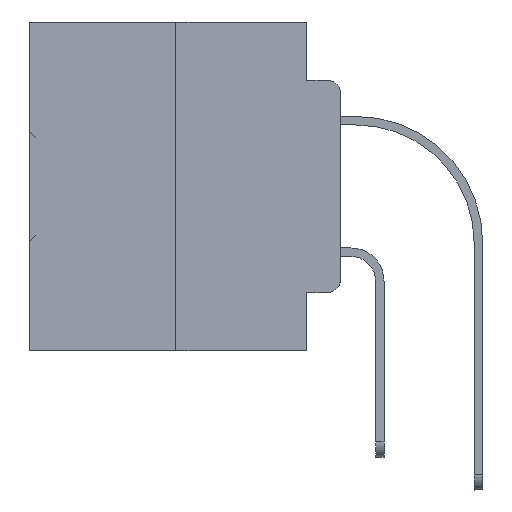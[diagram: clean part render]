
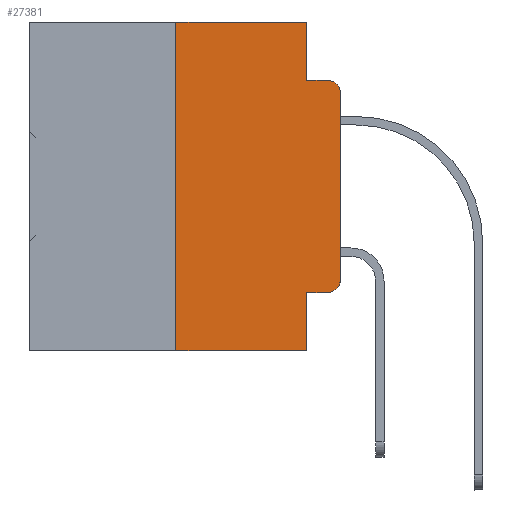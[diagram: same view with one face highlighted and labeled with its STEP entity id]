
A CAD part, left-side view. The second image highlights one B-rep face of the part: STEP entity #27381.
In plain terms, the highlighted planar face has unit normal (-1, 0, 0).
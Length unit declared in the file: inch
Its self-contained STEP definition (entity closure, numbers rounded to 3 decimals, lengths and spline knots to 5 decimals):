
#19 = AXIS2_PLACEMENT_3D ( 'NONE', #2751, #27768, #36520 ) ;
#204 = EDGE_CURVE ( 'NONE', #30506, #1603, #18048, .T. ) ;
#694 = EDGE_CURVE ( 'NONE', #7196, #11373, #11854, .T. ) ;
#994 = LINE ( 'NONE', #1771, #31194 ) ;
#1603 = VERTEX_POINT ( 'NONE', #6461 ) ;
#1771 = CARTESIAN_POINT ( 'NONE',  ( 0., 0.473, 0. ) ) ;
#2020 = ORIENTED_EDGE ( 'NONE', *, *, #25787, .T. ) ;
#2518 = CARTESIAN_POINT ( 'NONE',  ( 0., 0.051, -0.0885 ) ) ;
#2581 = CARTESIAN_POINT ( 'NONE',  ( 0., 0., -0.3915 ) ) ;
#2751 = CARTESIAN_POINT ( 'NONE',  ( 0., 0.02, -0.1085 ) ) ;
#2924 = AXIS2_PLACEMENT_3D ( 'NONE', #39070, #3511, #15623 ) ;
#3511 = DIRECTION ( 'NONE',  ( -1., 0., 0. ) ) ;
#3796 = VECTOR ( 'NONE', #8184, 39.37008 ) ;
#3831 = CARTESIAN_POINT ( 'NONE',  ( 0., 0.02, -0.0885 ) ) ;
#5427 = VERTEX_POINT ( 'NONE', #3831 ) ;
#5601 = CARTESIAN_POINT ( 'NONE',  ( 0., 0.25, -0.5 ) ) ;
#6103 = CARTESIAN_POINT ( 'NONE',  ( 0., 0.051, 0. ) ) ;
#6461 = CARTESIAN_POINT ( 'NONE',  ( 0., 0., -0.1085 ) ) ;
#6709 = LINE ( 'NONE', #9896, #29481 ) ;
#7196 = VERTEX_POINT ( 'NONE', #13130 ) ;
#7293 = EDGE_LOOP ( 'NONE', ( #32041, #2020, #10279, #28550, #11513, #8121, #36256, #29615, #19714, #32729 ) ) ;
#8121 = ORIENTED_EDGE ( 'NONE', *, *, #8737, .F. ) ;
#8184 = DIRECTION ( 'NONE',  ( 0., 0., -1. ) ) ;
#8220 = VERTEX_POINT ( 'NONE', #26532 ) ;
#8737 = EDGE_CURVE ( 'NONE', #34902, #21432, #23320, .T. ) ;
#8749 = CARTESIAN_POINT ( 'NONE',  ( 0., 0.473, 0. ) ) ;
#8863 = CARTESIAN_POINT ( 'NONE',  ( 0., 0.051, -0.4115 ) ) ;
#9896 = CARTESIAN_POINT ( 'NONE',  ( 0., 0.473, -0.5 ) ) ;
#10279 = ORIENTED_EDGE ( 'NONE', *, *, #29222, .F. ) ;
#10692 = VECTOR ( 'NONE', #11707, 39.37008 ) ;
#10774 = VECTOR ( 'NONE', #14644, 39.37008 ) ;
#11373 = VERTEX_POINT ( 'NONE', #23570 ) ;
#11513 = ORIENTED_EDGE ( 'NONE', *, *, #32243, .F. ) ;
#11707 = DIRECTION ( 'NONE',  ( 0., 0., 1. ) ) ;
#11830 = VERTEX_POINT ( 'NONE', #22937 ) ;
#11854 = LINE ( 'NONE', #8863, #33545 ) ;
#13130 = CARTESIAN_POINT ( 'NONE',  ( 0., 0.051, -0.4115 ) ) ;
#14644 = DIRECTION ( 'NONE',  ( 0., -1., 0. ) ) ;
#14696 = EDGE_CURVE ( 'NONE', #34902, #8220, #6709, .T. ) ;
#15225 = DIRECTION ( 'NONE',  ( 0., 0., -1. ) ) ;
#15623 = DIRECTION ( 'NONE',  ( 0., 0., -1. ) ) ;
#15821 = DIRECTION ( 'NONE',  ( 0., -1., 0. ) ) ;
#16306 = VECTOR ( 'NONE', #37994, 39.37008 ) ;
#16906 = CIRCLE ( 'NONE', #2924, 0.02 ) ;
#18048 = LINE ( 'NONE', #24007, #10692 ) ;
#19714 = ORIENTED_EDGE ( 'NONE', *, *, #694, .T. ) ;
#20309 = VECTOR ( 'NONE', #15225, 39.37008 ) ;
#20626 = LINE ( 'NONE', #2518, #10774 ) ;
#21432 = VERTEX_POINT ( 'NONE', #30860 ) ;
#22937 = CARTESIAN_POINT ( 'NONE',  ( 0., 0.051, 0. ) ) ;
#23320 = LINE ( 'NONE', #35421, #16306 ) ;
#23570 = CARTESIAN_POINT ( 'NONE',  ( 0., 0.02, -0.4115 ) ) ;
#24007 = CARTESIAN_POINT ( 'NONE',  ( 0., 0., 0. ) ) ;
#25787 = EDGE_CURVE ( 'NONE', #1603, #5427, #34275, .T. ) ;
#26170 = DIRECTION ( 'NONE',  ( 0., -1., 0. ) ) ;
#26532 = CARTESIAN_POINT ( 'NONE',  ( 0., 0.051, -0.5 ) ) ;
#27197 = PLANE ( 'NONE',  #31227 ) ;
#27381 = ADVANCED_FACE ( 'NONE', ( #38926 ), #27197, .F. ) ;
#27768 = DIRECTION ( 'NONE',  ( -1., 0., 0. ) ) ;
#28550 = ORIENTED_EDGE ( 'NONE', *, *, #29347, .F. ) ;
#29222 = EDGE_CURVE ( 'NONE', #33421, #5427, #20626, .T. ) ;
#29347 = EDGE_CURVE ( 'NONE', #11830, #33421, #34094, .T. ) ;
#29417 = DIRECTION ( 'NONE',  ( 0., 0., -1. ) ) ;
#29481 = VECTOR ( 'NONE', #15821, 39.37008 ) ;
#29615 = ORIENTED_EDGE ( 'NONE', *, *, #30478, .F. ) ;
#30478 = EDGE_CURVE ( 'NONE', #7196, #8220, #35968, .T. ) ;
#30506 = VERTEX_POINT ( 'NONE', #2581 ) ;
#30656 = CARTESIAN_POINT ( 'NONE',  ( 0., 0.051, -0.0885 ) ) ;
#30860 = CARTESIAN_POINT ( 'NONE',  ( 0., 0.25, 0. ) ) ;
#31194 = VECTOR ( 'NONE', #31388, 39.37008 ) ;
#31227 = AXIS2_PLACEMENT_3D ( 'NONE', #8749, #35951, #29417 ) ;
#31388 = DIRECTION ( 'NONE',  ( 0., -1., 0. ) ) ;
#32041 = ORIENTED_EDGE ( 'NONE', *, *, #204, .T. ) ;
#32243 = EDGE_CURVE ( 'NONE', #21432, #11830, #994, .T. ) ;
#32729 = ORIENTED_EDGE ( 'NONE', *, *, #38869, .T. ) ;
#33421 = VERTEX_POINT ( 'NONE', #30656 ) ;
#33545 = VECTOR ( 'NONE', #26170, 39.37008 ) ;
#34094 = LINE ( 'NONE', #6103, #20309 ) ;
#34275 = CIRCLE ( 'NONE', #19, 0.02 ) ;
#34902 = VERTEX_POINT ( 'NONE', #5601 ) ;
#35421 = CARTESIAN_POINT ( 'NONE',  ( 0., 0.25, 0. ) ) ;
#35951 = DIRECTION ( 'NONE',  ( 1., 0., 0. ) ) ;
#35968 = LINE ( 'NONE', #39128, #3796 ) ;
#36256 = ORIENTED_EDGE ( 'NONE', *, *, #14696, .T. ) ;
#36520 = DIRECTION ( 'NONE',  ( 0., 0., -1. ) ) ;
#37994 = DIRECTION ( 'NONE',  ( 0., 0., 1. ) ) ;
#38869 = EDGE_CURVE ( 'NONE', #11373, #30506, #16906, .T. ) ;
#38926 = FACE_OUTER_BOUND ( 'NONE', #7293, .T. ) ;
#39070 = CARTESIAN_POINT ( 'NONE',  ( 0., 0.02, -0.3915 ) ) ;
#39128 = CARTESIAN_POINT ( 'NONE',  ( 0., 0.051, 0. ) ) ;
